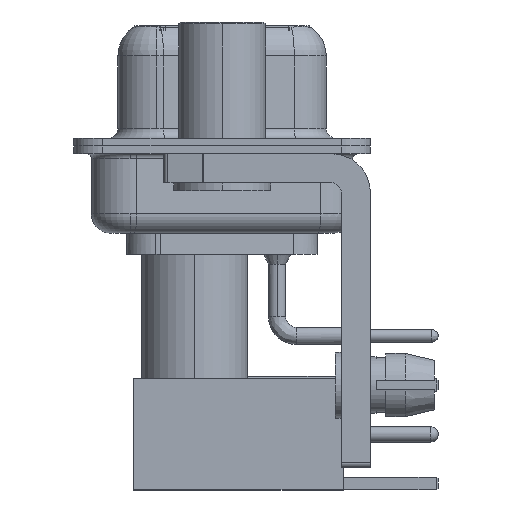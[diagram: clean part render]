
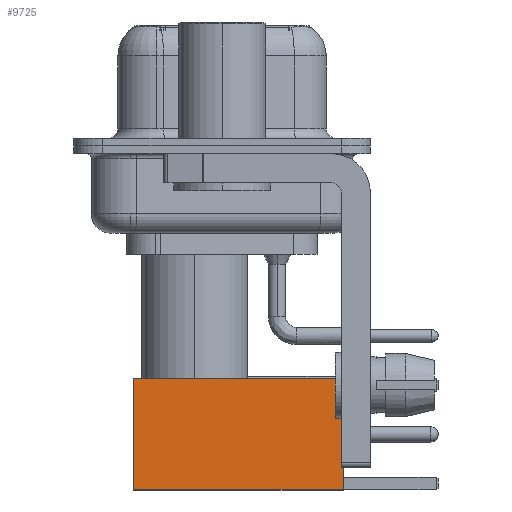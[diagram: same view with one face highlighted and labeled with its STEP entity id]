
A CAD part, left-side view. The second image highlights one B-rep face of the part: STEP entity #9725.
In plain terms, the highlighted face is planar.
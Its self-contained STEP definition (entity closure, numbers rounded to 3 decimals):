
#336 = CARTESIAN_POINT ( 'NONE',  ( -2.875, 2.875, 0. ) ) ;
#862 = EDGE_CURVE ( 'NONE', #33653, #39265, #1664, .T. ) ;
#1354 = LINE ( 'NONE', #20856, #13434 ) ;
#1583 = DIRECTION ( 'NONE',  ( 0., 0., 1. ) ) ;
#1664 = LINE ( 'NONE', #11528, #8983 ) ;
#3248 = CARTESIAN_POINT ( 'NONE',  ( 0., 2.875, 10.82 ) ) ;
#6110 = ORIENTED_EDGE ( 'NONE', *, *, #26238, .F. ) ;
#8563 = PLANE ( 'NONE',  #34987 ) ;
#8983 = VECTOR ( 'NONE', #32893, 1000. ) ;
#9725 = ADVANCED_FACE ( 'NONE', ( #11840 ), #8563, .T. ) ;
#9965 = VERTEX_POINT ( 'NONE', #16155 ) ;
#11238 = CARTESIAN_POINT ( 'NONE',  ( 2.875, 2.875, 0. ) ) ;
#11528 = CARTESIAN_POINT ( 'NONE',  ( 0., 2.875, 0. ) ) ;
#11840 = FACE_OUTER_BOUND ( 'NONE', #14483, .T. ) ;
#13029 = VERTEX_POINT ( 'NONE', #17886 ) ;
#13434 = VECTOR ( 'NONE', #16785, 1000. ) ;
#14483 = EDGE_LOOP ( 'NONE', ( #21145, #35482, #38802, #6110 ) ) ;
#16155 = CARTESIAN_POINT ( 'NONE',  ( 2.875, 2.875, 10.82 ) ) ;
#16785 = DIRECTION ( 'NONE',  ( 0., 0., -1. ) ) ;
#17886 = CARTESIAN_POINT ( 'NONE',  ( -2.875, 2.875, 10.82 ) ) ;
#18454 = DIRECTION ( 'NONE',  ( -1., 0., 0. ) ) ;
#20001 = EDGE_CURVE ( 'NONE', #9965, #33653, #1354, .T. ) ;
#20856 = CARTESIAN_POINT ( 'NONE',  ( 2.875, 2.875, 0. ) ) ;
#21145 = ORIENTED_EDGE ( 'NONE', *, *, #20001, .T. ) ;
#22207 = EDGE_CURVE ( 'NONE', #13029, #39265, #31563, .T. ) ;
#23419 = CARTESIAN_POINT ( 'NONE',  ( 2.875, 2.875, 0. ) ) ;
#26238 = EDGE_CURVE ( 'NONE', #9965, #13029, #37991, .T. ) ;
#27454 = DIRECTION ( 'NONE',  ( 0., 1., 0. ) ) ;
#28485 = DIRECTION ( 'NONE',  ( 0., 0., -1. ) ) ;
#28681 = CARTESIAN_POINT ( 'NONE',  ( -2.875, 2.875, 0. ) ) ;
#30985 = VECTOR ( 'NONE', #28485, 1000. ) ;
#31198 = VECTOR ( 'NONE', #18454, 1000. ) ;
#31563 = LINE ( 'NONE', #28681, #30985 ) ;
#32893 = DIRECTION ( 'NONE',  ( -1., 0., 0. ) ) ;
#33653 = VERTEX_POINT ( 'NONE', #23419 ) ;
#34987 = AXIS2_PLACEMENT_3D ( 'NONE', #11238, #27454, #1583 ) ;
#35482 = ORIENTED_EDGE ( 'NONE', *, *, #862, .T. ) ;
#37991 = LINE ( 'NONE', #3248, #31198 ) ;
#38802 = ORIENTED_EDGE ( 'NONE', *, *, #22207, .F. ) ;
#39265 = VERTEX_POINT ( 'NONE', #336 ) ;
